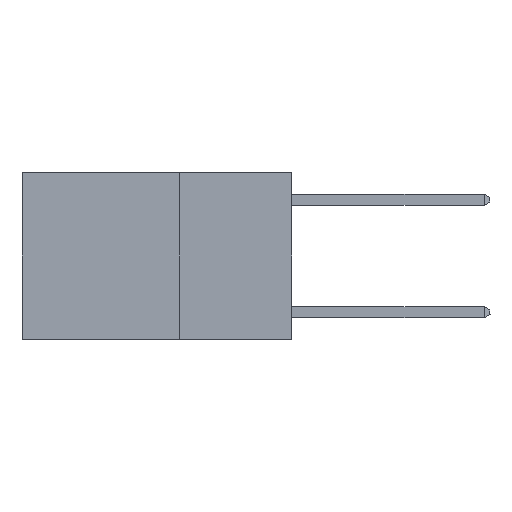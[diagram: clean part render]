
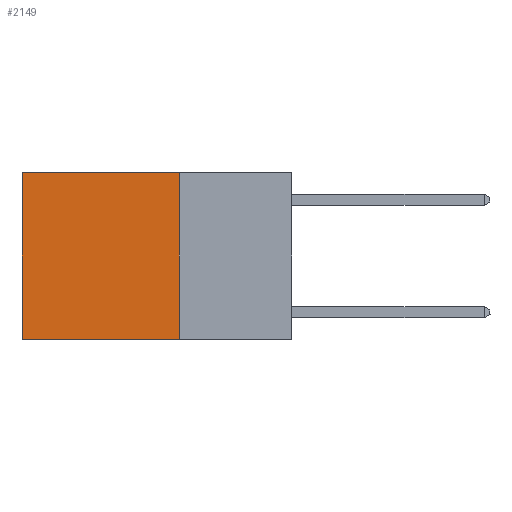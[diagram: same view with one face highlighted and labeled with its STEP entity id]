
A CAD part, left-side view. The second image highlights one B-rep face of the part: STEP entity #2149.
In plain terms, the highlighted planar face has unit normal (-1, 0, 0).
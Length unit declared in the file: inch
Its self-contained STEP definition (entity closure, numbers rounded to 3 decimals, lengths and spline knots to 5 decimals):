
#70 = EDGE_CURVE ( 'NONE', #13898, #15844, #12174, .T. ) ;
#2111 = DIRECTION ( 'NONE',  ( 0., 1., 0. ) ) ;
#2145 = LINE ( 'NONE', #10969, #17627 ) ;
#2149 = ADVANCED_FACE ( 'NONE', ( #4345 ), #14715, .F. ) ;
#3087 = CARTESIAN_POINT ( 'NONE',  ( 0.2625, 0.25, 0. ) ) ;
#3286 = ORIENTED_EDGE ( 'NONE', *, *, #4019, .F. ) ;
#3566 = ORIENTED_EDGE ( 'NONE', *, *, #6175, .T. ) ;
#4018 = VECTOR ( 'NONE', #16951, 39.37008 ) ;
#4019 = EDGE_CURVE ( 'NONE', #10146, #13898, #2145, .T. ) ;
#4345 = FACE_OUTER_BOUND ( 'NONE', #5231, .T. ) ;
#4390 = ORIENTED_EDGE ( 'NONE', *, *, #70, .F. ) ;
#5144 = VERTEX_POINT ( 'NONE', #17311 ) ;
#5231 = EDGE_LOOP ( 'NONE', ( #3566, #4390, #3286, #15129 ) ) ;
#5326 = LINE ( 'NONE', #18374, #16371 ) ;
#6175 = EDGE_CURVE ( 'NONE', #5144, #15844, #12460, .T. ) ;
#6751 = DIRECTION ( 'NONE',  ( 0., 1., 0. ) ) ;
#7395 = CARTESIAN_POINT ( 'NONE',  ( 0.2625, 0.6, -0.37 ) ) ;
#8713 = DIRECTION ( 'NONE',  ( 0., 0., -1. ) ) ;
#9259 = DIRECTION ( 'NONE',  ( 0., 0., -1. ) ) ;
#9984 = AXIS2_PLACEMENT_3D ( 'NONE', #13092, #15968, #8713 ) ;
#10146 = VERTEX_POINT ( 'NONE', #3087 ) ;
#10969 = CARTESIAN_POINT ( 'NONE',  ( 0.2625, 0.25, 0. ) ) ;
#12174 = LINE ( 'NONE', #18089, #12277 ) ;
#12277 = VECTOR ( 'NONE', #2111, 39.37008 ) ;
#12460 = LINE ( 'NONE', #15331, #4018 ) ;
#13092 = CARTESIAN_POINT ( 'NONE',  ( 0.2625, 0.25, 0. ) ) ;
#13898 = VERTEX_POINT ( 'NONE', #14201 ) ;
#14201 = CARTESIAN_POINT ( 'NONE',  ( 0.2625, 0.25, -0.37 ) ) ;
#14715 = PLANE ( 'NONE',  #9984 ) ;
#15129 = ORIENTED_EDGE ( 'NONE', *, *, #18645, .T. ) ;
#15331 = CARTESIAN_POINT ( 'NONE',  ( 0.2625, 0.6, 0. ) ) ;
#15844 = VERTEX_POINT ( 'NONE', #7395 ) ;
#15968 = DIRECTION ( 'NONE',  ( 1., 0., 0. ) ) ;
#16371 = VECTOR ( 'NONE', #6751, 39.37008 ) ;
#16951 = DIRECTION ( 'NONE',  ( 0., 0., -1. ) ) ;
#17311 = CARTESIAN_POINT ( 'NONE',  ( 0.2625, 0.6, 0. ) ) ;
#17627 = VECTOR ( 'NONE', #9259, 39.37008 ) ;
#18089 = CARTESIAN_POINT ( 'NONE',  ( 0.2625, 0.25, -0.37 ) ) ;
#18374 = CARTESIAN_POINT ( 'NONE',  ( 0.2625, 0.25, 0. ) ) ;
#18645 = EDGE_CURVE ( 'NONE', #10146, #5144, #5326, .T. ) ;
